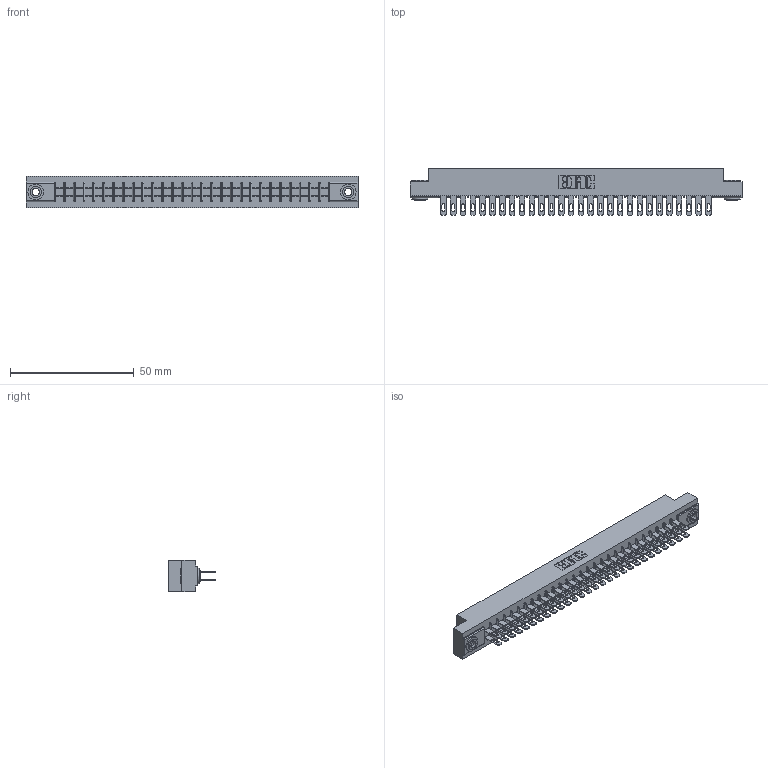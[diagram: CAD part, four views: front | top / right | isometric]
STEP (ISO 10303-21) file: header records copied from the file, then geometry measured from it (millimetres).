
FILE_DESCRIPTION (( 'STEP AP203' ), '1' );
FILE_NAME ('305-056-500-203.STEP', '2019-09-09T23:25:51', ( '' ), ( '' ), 'SwSTEP 2.0', 'SolidWorks 2016', '' );
FILE_SCHEMA (( 'CONFIG_CONTROL_DESIGN' ));
Length unit declared in the file: inch
Products named in the file (4): 345-250-002_345-250-002-102; 305-056-500-203; 305 Part_.156 Dia; 305-290-001_500
Assembly tree (59 placements, depth 2):
  305-056-500-203
    305 Part_.156 Dia
    305-290-001_500  x56
    345-250-002_345-250-002-102  x2
Bounding box: 133.96 x 18.85 x 12.7 mm (x, y, z)
Volume: 14061.6 mm3; surface area: 18922.7 mm2
Topology: 59 solids, 59 shells, 2968 faces, 8464 edges, 5488 vertices
Faces by surface type: plane 1660, cylinder 1188, sphere 112, cone 8
Entity records: 33108 total; most frequent: CARTESIAN_POINT 5459, ORIENTED_EDGE 5408, DIRECTION 5310, EDGE_CURVE 2704, LINE 2160, VECTOR 2160, VERTEX_POINT 1724, AXIS2_PLACEMENT_3D 1575
